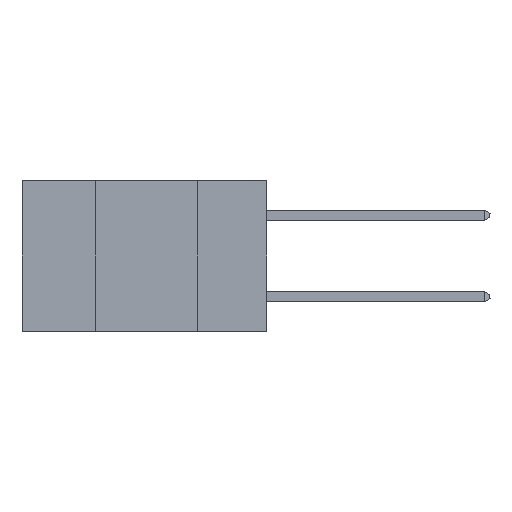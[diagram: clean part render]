
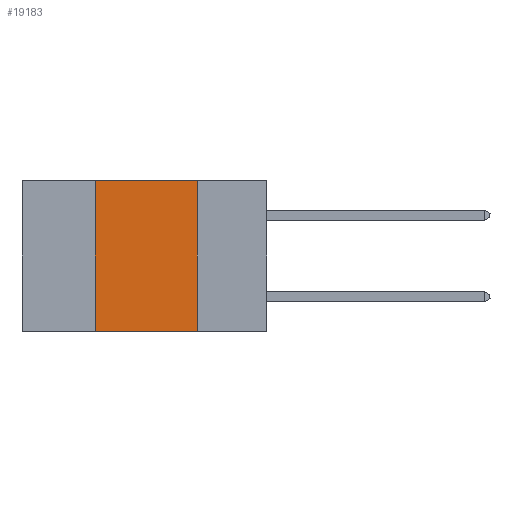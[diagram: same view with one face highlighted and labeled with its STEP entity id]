
A CAD part, left-side view. The second image highlights one B-rep face of the part: STEP entity #19183.
In plain terms, the highlighted planar face has unit normal (-1, 0, 0).
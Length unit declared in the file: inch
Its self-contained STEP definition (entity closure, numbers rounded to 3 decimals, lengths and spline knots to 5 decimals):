
#354 = DIRECTION ( 'NONE',  ( 1., 0., 0. ) ) ;
#949 = ORIENTED_EDGE ( 'NONE', *, *, #12743, .F. ) ;
#1012 = LINE ( 'NONE', #4507, #14501 ) ;
#1095 = LINE ( 'NONE', #20435, #13188 ) ;
#2644 = DIRECTION ( 'NONE',  ( 0., -1., 0. ) ) ;
#4507 = CARTESIAN_POINT ( 'NONE',  ( 0., 0.17, 0. ) ) ;
#5436 = ORIENTED_EDGE ( 'NONE', *, *, #15420, .F. ) ;
#7209 = LINE ( 'NONE', #20300, #29903 ) ;
#7576 = EDGE_CURVE ( 'NONE', #38246, #35116, #13929, .T. ) ;
#9479 = CARTESIAN_POINT ( 'NONE',  ( 0., 0.42, 0. ) ) ;
#12047 = CARTESIAN_POINT ( 'NONE',  ( 0., 0.6, 0. ) ) ;
#12438 = DIRECTION ( 'NONE',  ( 0., 0., -1. ) ) ;
#12743 = EDGE_CURVE ( 'NONE', #23384, #31690, #1012, .T. ) ;
#12833 = AXIS2_PLACEMENT_3D ( 'NONE', #12047, #354, #12438 ) ;
#13188 = VECTOR ( 'NONE', #38250, 39.37008 ) ;
#13461 = DIRECTION ( 'NONE',  ( 0., 0., -1. ) ) ;
#13929 = LINE ( 'NONE', #9479, #14388 ) ;
#14388 = VECTOR ( 'NONE', #27000, 39.37008 ) ;
#14501 = VECTOR ( 'NONE', #13461, 39.37008 ) ;
#15420 = EDGE_CURVE ( 'NONE', #35116, #23384, #1095, .T. ) ;
#17235 = ORIENTED_EDGE ( 'NONE', *, *, #37159, .T. ) ;
#19183 = ADVANCED_FACE ( 'NONE', ( #36886 ), #31841, .F. ) ;
#19323 = CARTESIAN_POINT ( 'NONE',  ( 0., 0.42, -0.37 ) ) ;
#20300 = CARTESIAN_POINT ( 'NONE',  ( 0., 0.6, -0.37 ) ) ;
#20435 = CARTESIAN_POINT ( 'NONE',  ( 0., 0.6, 0. ) ) ;
#23384 = VERTEX_POINT ( 'NONE', #24935 ) ;
#24935 = CARTESIAN_POINT ( 'NONE',  ( 0., 0.17, 0. ) ) ;
#27000 = DIRECTION ( 'NONE',  ( 0., 0., 1. ) ) ;
#28678 = EDGE_LOOP ( 'NONE', ( #949, #5436, #33400, #17235 ) ) ;
#29903 = VECTOR ( 'NONE', #2644, 39.37008 ) ;
#31690 = VERTEX_POINT ( 'NONE', #34985 ) ;
#31841 = PLANE ( 'NONE',  #12833 ) ;
#33400 = ORIENTED_EDGE ( 'NONE', *, *, #7576, .F. ) ;
#34859 = CARTESIAN_POINT ( 'NONE',  ( 0., 0.42, 0. ) ) ;
#34985 = CARTESIAN_POINT ( 'NONE',  ( 0., 0.17, -0.37 ) ) ;
#35116 = VERTEX_POINT ( 'NONE', #34859 ) ;
#36886 = FACE_OUTER_BOUND ( 'NONE', #28678, .T. ) ;
#37159 = EDGE_CURVE ( 'NONE', #38246, #31690, #7209, .T. ) ;
#38246 = VERTEX_POINT ( 'NONE', #19323 ) ;
#38250 = DIRECTION ( 'NONE',  ( 0., -1., 0. ) ) ;
